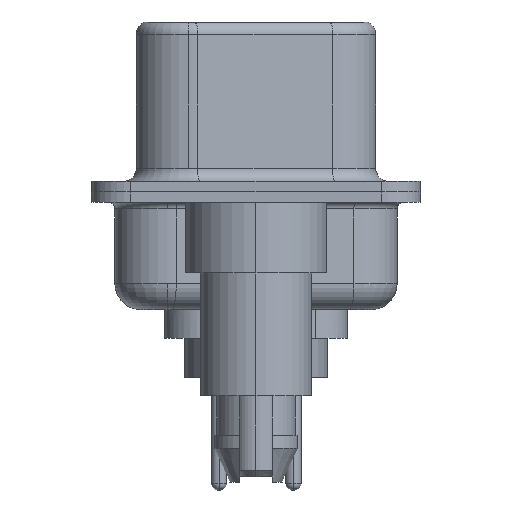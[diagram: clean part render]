
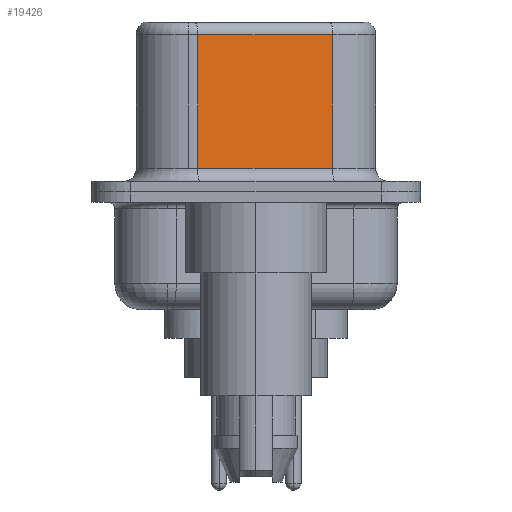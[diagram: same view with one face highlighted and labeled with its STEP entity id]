
A CAD part, left-side view. The second image highlights one B-rep face of the part: STEP entity #19426.
In plain terms, the highlighted planar face has unit normal (-0.985, -0.174, 0).
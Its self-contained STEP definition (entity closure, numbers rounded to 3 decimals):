
#542 = VERTEX_POINT ( 'NONE', #926 ) ;
#926 = CARTESIAN_POINT ( 'NONE',  ( 3.675, 2.233, 6.02 ) ) ;
#1145 = CARTESIAN_POINT ( 'NONE',  ( 4.585, -2.927, 6.52 ) ) ;
#1259 = ORIENTED_EDGE ( 'NONE', *, *, #5163, .T. ) ;
#1377 = VERTEX_POINT ( 'NONE', #17530 ) ;
#1793 = CARTESIAN_POINT ( 'NONE',  ( 4.585, -2.927, 6.02 ) ) ;
#2673 = DIRECTION ( 'NONE',  ( 0.174, -0.985, 0. ) ) ;
#3054 = CARTESIAN_POINT ( 'NONE',  ( 4.585, -2.927, 6.52 ) ) ;
#3557 = LINE ( 'NONE', #1145, #16708 ) ;
#4792 = DIRECTION ( 'NONE',  ( -0.174, 0.985, 0. ) ) ;
#5163 = EDGE_CURVE ( 'NONE', #7014, #542, #15390, .T. ) ;
#6125 = VECTOR ( 'NONE', #2673, 1000. ) ;
#6282 = VECTOR ( 'NONE', #6966, 1000. ) ;
#6686 = FACE_OUTER_BOUND ( 'NONE', #8612, .T. ) ;
#6966 = DIRECTION ( 'NONE',  ( -0.174, 0.985, 0. ) ) ;
#7014 = VERTEX_POINT ( 'NONE', #18033 ) ;
#8148 = ORIENTED_EDGE ( 'NONE', *, *, #10340, .T. ) ;
#8177 = PLANE ( 'NONE',  #22066 ) ;
#8612 = EDGE_LOOP ( 'NONE', ( #19132, #1259, #8148, #14103 ) ) ;
#9105 = EDGE_CURVE ( 'NONE', #16467, #1377, #9111, .T. ) ;
#9111 = LINE ( 'NONE', #14649, #6125 ) ;
#10340 = EDGE_CURVE ( 'NONE', #542, #16467, #21114, .T. ) ;
#10772 = EDGE_CURVE ( 'NONE', #7014, #1377, #3557, .T. ) ;
#11194 = CARTESIAN_POINT ( 'NONE',  ( 3.675, 2.233, 6.52 ) ) ;
#11355 = DIRECTION ( 'NONE',  ( 0., 0., -1. ) ) ;
#11946 = VECTOR ( 'NONE', #19838, 1000. ) ;
#14103 = ORIENTED_EDGE ( 'NONE', *, *, #9105, .T. ) ;
#14649 = CARTESIAN_POINT ( 'NONE',  ( 4.585, -2.927, 0.9 ) ) ;
#15035 = DIRECTION ( 'NONE',  ( 0.985, 0.174, 0. ) ) ;
#15390 = LINE ( 'NONE', #1793, #6282 ) ;
#16467 = VERTEX_POINT ( 'NONE', #18461 ) ;
#16708 = VECTOR ( 'NONE', #11355, 1000. ) ;
#17530 = CARTESIAN_POINT ( 'NONE',  ( 4.585, -2.927, 0.9 ) ) ;
#18033 = CARTESIAN_POINT ( 'NONE',  ( 4.585, -2.927, 6.02 ) ) ;
#18461 = CARTESIAN_POINT ( 'NONE',  ( 3.675, 2.233, 0.9 ) ) ;
#19132 = ORIENTED_EDGE ( 'NONE', *, *, #10772, .F. ) ;
#19426 = ADVANCED_FACE ( 'NONE', ( #6686 ), #8177, .F. ) ;
#19838 = DIRECTION ( 'NONE',  ( 0., 0., -1. ) ) ;
#21114 = LINE ( 'NONE', #11194, #11946 ) ;
#22066 = AXIS2_PLACEMENT_3D ( 'NONE', #3054, #15035, #4792 ) ;
